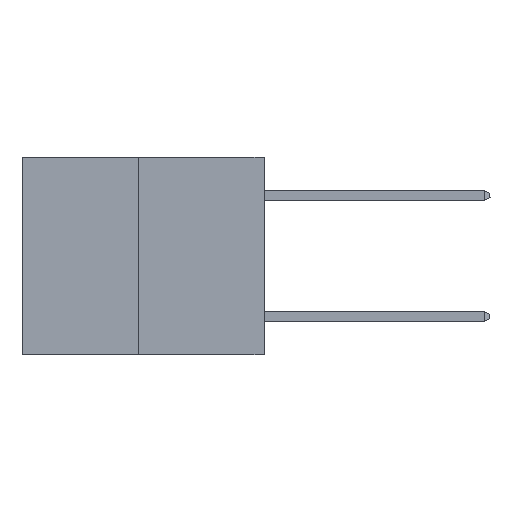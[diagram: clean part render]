
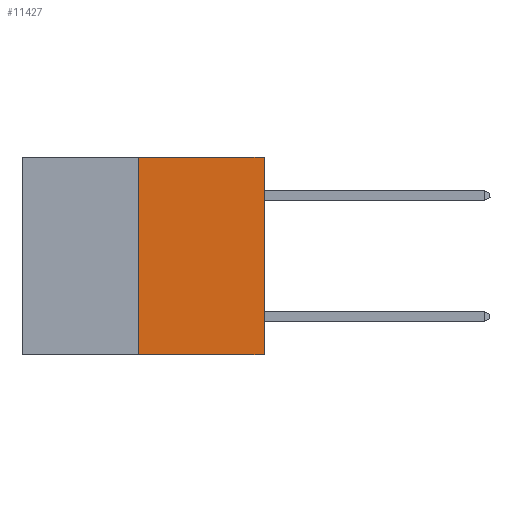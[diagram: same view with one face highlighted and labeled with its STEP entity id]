
A CAD part, left-side view. The second image highlights one B-rep face of the part: STEP entity #11427.
In plain terms, the highlighted planar face has unit normal (-1, 0, 0).
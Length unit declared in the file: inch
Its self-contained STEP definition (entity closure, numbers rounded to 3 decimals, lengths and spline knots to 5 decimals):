
#365 = AXIS2_PLACEMENT_3D ( 'NONE', #27180, #9812, #3527 ) ;
#418 = CARTESIAN_POINT ( 'NONE',  ( 0., 0.6, -0.49 ) ) ;
#1178 = CARTESIAN_POINT ( 'NONE',  ( 0., 0.312, -0.49 ) ) ;
#1440 = CARTESIAN_POINT ( 'NONE',  ( 0., 0., 0. ) ) ;
#2391 = VECTOR ( 'NONE', #4809, 39.37008 ) ;
#3295 = ORIENTED_EDGE ( 'NONE', *, *, #21144, .T. ) ;
#3527 = DIRECTION ( 'NONE',  ( 0., 0., -1. ) ) ;
#3906 = VECTOR ( 'NONE', #25387, 39.37008 ) ;
#4531 = DIRECTION ( 'NONE',  ( 0., -1., 0. ) ) ;
#4643 = LINE ( 'NONE', #418, #8289 ) ;
#4809 = DIRECTION ( 'NONE',  ( 0., -1., 0. ) ) ;
#5242 = LINE ( 'NONE', #10374, #3906 ) ;
#6133 = EDGE_CURVE ( 'NONE', #21103, #17972, #5242, .T. ) ;
#8224 = CARTESIAN_POINT ( 'NONE',  ( 0., 0.312, 0. ) ) ;
#8289 = VECTOR ( 'NONE', #4531, 39.37008 ) ;
#9360 = ORIENTED_EDGE ( 'NONE', *, *, #6133, .F. ) ;
#9812 = DIRECTION ( 'NONE',  ( 1., 0., 0. ) ) ;
#9909 = EDGE_CURVE ( 'NONE', #17972, #12224, #26837, .T. ) ;
#10374 = CARTESIAN_POINT ( 'NONE',  ( 0., 0.312, -0.49 ) ) ;
#11427 = ADVANCED_FACE ( 'NONE', ( #17713 ), #12101, .F. ) ;
#12101 = PLANE ( 'NONE',  #365 ) ;
#12153 = ORIENTED_EDGE ( 'NONE', *, *, #25242, .T. ) ;
#12224 = VERTEX_POINT ( 'NONE', #18938 ) ;
#15938 = LINE ( 'NONE', #1440, #26647 ) ;
#17351 = CARTESIAN_POINT ( 'NONE',  ( 0., 0., -0.49 ) ) ;
#17713 = FACE_OUTER_BOUND ( 'NONE', #21017, .T. ) ;
#17972 = VERTEX_POINT ( 'NONE', #8224 ) ;
#18938 = CARTESIAN_POINT ( 'NONE',  ( 0., 0., 0. ) ) ;
#20027 = CARTESIAN_POINT ( 'NONE',  ( 0., 0.6, 0. ) ) ;
#20861 = VERTEX_POINT ( 'NONE', #17351 ) ;
#21017 = EDGE_LOOP ( 'NONE', ( #9360, #12153, #3295, #24622 ) ) ;
#21103 = VERTEX_POINT ( 'NONE', #1178 ) ;
#21144 = EDGE_CURVE ( 'NONE', #20861, #12224, #15938, .T. ) ;
#22727 = DIRECTION ( 'NONE',  ( 0., 0., 1. ) ) ;
#24622 = ORIENTED_EDGE ( 'NONE', *, *, #9909, .F. ) ;
#25242 = EDGE_CURVE ( 'NONE', #21103, #20861, #4643, .T. ) ;
#25387 = DIRECTION ( 'NONE',  ( 0., 0., 1. ) ) ;
#26647 = VECTOR ( 'NONE', #22727, 39.37008 ) ;
#26837 = LINE ( 'NONE', #20027, #2391 ) ;
#27180 = CARTESIAN_POINT ( 'NONE',  ( 0., 0.6, 0. ) ) ;
